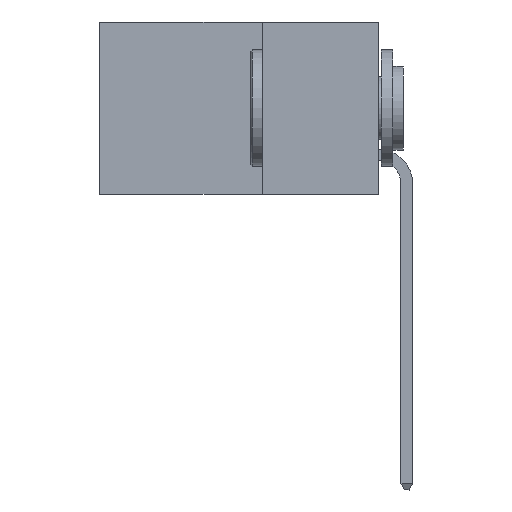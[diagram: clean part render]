
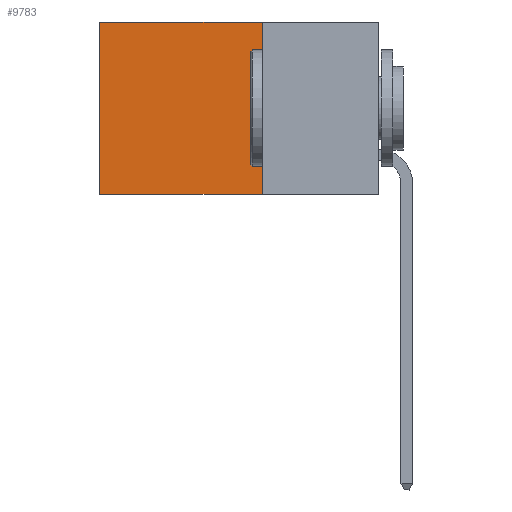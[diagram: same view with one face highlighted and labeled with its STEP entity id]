
A CAD part, left-side view. The second image highlights one B-rep face of the part: STEP entity #9783.
In plain terms, the highlighted planar face has unit normal (-1, 0, 0).
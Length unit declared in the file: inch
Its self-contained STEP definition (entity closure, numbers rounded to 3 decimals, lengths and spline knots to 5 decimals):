
#571 = LINE ( 'NONE', #15837, #7029 ) ;
#625 = PLANE ( 'NONE',  #5213 ) ;
#787 = DIRECTION ( 'NONE',  ( 0., 0., -1. ) ) ;
#874 = CARTESIAN_POINT ( 'NONE',  ( 0.2615, 0.25, -0.37 ) ) ;
#1891 = CARTESIAN_POINT ( 'NONE',  ( 0.2615, 0.25, -0.37 ) ) ;
#2097 = DIRECTION ( 'NONE',  ( 0., 1., 0. ) ) ;
#2510 = VECTOR ( 'NONE', #787, 39.37008 ) ;
#3171 = DIRECTION ( 'NONE',  ( 0., 0., -1. ) ) ;
#3482 = CARTESIAN_POINT ( 'NONE',  ( 0.2615, 0.25, -0.37 ) ) ;
#3500 = VERTEX_POINT ( 'NONE', #10870 ) ;
#4181 = FACE_OUTER_BOUND ( 'NONE', #11879, .T. ) ;
#4430 = LINE ( 'NONE', #1891, #15235 ) ;
#4944 = CARTESIAN_POINT ( 'NONE',  ( 0.2615, 0.25, 0. ) ) ;
#5213 = AXIS2_PLACEMENT_3D ( 'NONE', #11722, #9318, #3171 ) ;
#5670 = VECTOR ( 'NONE', #2097, 39.37008 ) ;
#6231 = VERTEX_POINT ( 'NONE', #3482 ) ;
#6921 = DIRECTION ( 'NONE',  ( 0., 0., -1. ) ) ;
#6936 = EDGE_CURVE ( 'NONE', #7757, #6231, #14579, .T. ) ;
#7029 = VECTOR ( 'NONE', #6921, 39.37008 ) ;
#7325 = ORIENTED_EDGE ( 'NONE', *, *, #8539, .T. ) ;
#7757 = VERTEX_POINT ( 'NONE', #4944 ) ;
#7993 = ORIENTED_EDGE ( 'NONE', *, *, #10672, .T. ) ;
#8539 = EDGE_CURVE ( 'NONE', #7757, #15574, #13420, .T. ) ;
#9318 = DIRECTION ( 'NONE',  ( 1., 0., 0. ) ) ;
#9408 = EDGE_CURVE ( 'NONE', #6231, #3500, #4430, .T. ) ;
#9783 = ADVANCED_FACE ( 'NONE', ( #4181 ), #625, .F. ) ;
#10672 = EDGE_CURVE ( 'NONE', #15574, #3500, #571, .T. ) ;
#10870 = CARTESIAN_POINT ( 'NONE',  ( 0.2615, 0.6, -0.37 ) ) ;
#11722 = CARTESIAN_POINT ( 'NONE',  ( 0.2615, 0.25, -0.37 ) ) ;
#11809 = ORIENTED_EDGE ( 'NONE', *, *, #6936, .F. ) ;
#11879 = EDGE_LOOP ( 'NONE', ( #7993, #15902, #11809, #7325 ) ) ;
#13420 = LINE ( 'NONE', #16135, #5670 ) ;
#14285 = DIRECTION ( 'NONE',  ( 0., 1., 0. ) ) ;
#14579 = LINE ( 'NONE', #874, #2510 ) ;
#15235 = VECTOR ( 'NONE', #14285, 39.37008 ) ;
#15574 = VERTEX_POINT ( 'NONE', #16031 ) ;
#15837 = CARTESIAN_POINT ( 'NONE',  ( 0.2615, 0.6, -0.37 ) ) ;
#15902 = ORIENTED_EDGE ( 'NONE', *, *, #9408, .F. ) ;
#16031 = CARTESIAN_POINT ( 'NONE',  ( 0.2615, 0.6, 0. ) ) ;
#16135 = CARTESIAN_POINT ( 'NONE',  ( 0.2615, 0.25, 0. ) ) ;
